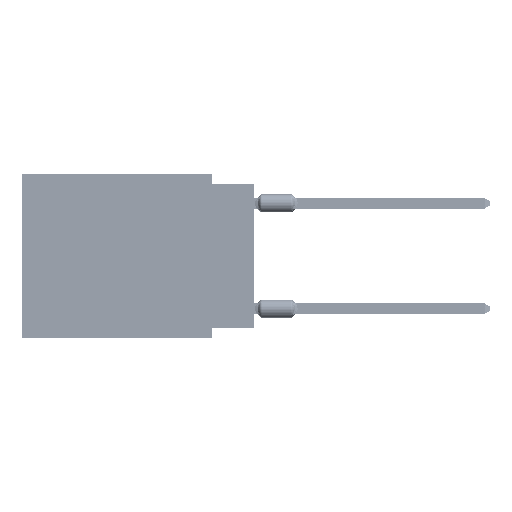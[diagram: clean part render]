
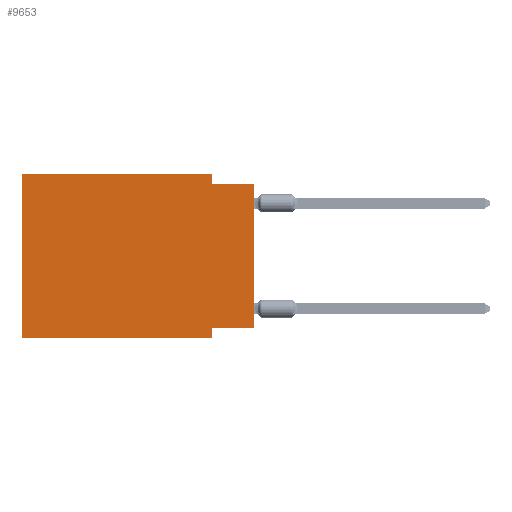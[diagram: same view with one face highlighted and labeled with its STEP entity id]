
A CAD part, left-side view. The second image highlights one B-rep face of the part: STEP entity #9653.
In plain terms, the highlighted planar face has unit normal (-1, 0, 0).
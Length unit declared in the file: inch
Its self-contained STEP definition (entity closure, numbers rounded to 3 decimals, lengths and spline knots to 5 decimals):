
#1042 = PLANE ( 'NONE',  #41379 ) ;
#1323 = LINE ( 'NONE', #72326, #17636 ) ;
#2230 = VECTOR ( 'NONE', #40724, 39.37008 ) ;
#2346 = VERTEX_POINT ( 'NONE', #14057 ) ;
#6202 = ORIENTED_EDGE ( 'NONE', *, *, #41951, .F. ) ;
#7195 = LINE ( 'NONE', #78625, #16957 ) ;
#7771 = VERTEX_POINT ( 'NONE', #80201 ) ;
#7961 = LINE ( 'NONE', #38356, #2230 ) ;
#8092 = VERTEX_POINT ( 'NONE', #33844 ) ;
#9653 = ADVANCED_FACE ( 'NONE', ( #72862 ), #1042, .F. ) ;
#11937 = VERTEX_POINT ( 'NONE', #57361 ) ;
#12796 = LINE ( 'NONE', #76288, #73460 ) ;
#13601 = EDGE_CURVE ( 'NONE', #22929, #8092, #1323, .T. ) ;
#14057 = CARTESIAN_POINT ( 'NONE',  ( 0., 0.55, 0. ) ) ;
#15280 = CARTESIAN_POINT ( 'NONE',  ( 0., 0.55, 0. ) ) ;
#15868 = CARTESIAN_POINT ( 'NONE',  ( 0., 0.1, -0.39 ) ) ;
#16957 = VECTOR ( 'NONE', #77391, 39.37008 ) ;
#17636 = VECTOR ( 'NONE', #26919, 39.37008 ) ;
#21873 = LINE ( 'NONE', #29428, #29114 ) ;
#22428 = EDGE_LOOP ( 'NONE', ( #67440, #48752, #23538, #30403, #28441, #42413, #27757, #6202 ) ) ;
#22727 = VERTEX_POINT ( 'NONE', #46917 ) ;
#22929 = VERTEX_POINT ( 'NONE', #25560 ) ;
#23538 = ORIENTED_EDGE ( 'NONE', *, *, #61757, .F. ) ;
#24059 = LINE ( 'NONE', #50974, #32996 ) ;
#25560 = CARTESIAN_POINT ( 'NONE',  ( 0., 0., -0.365 ) ) ;
#26069 = VECTOR ( 'NONE', #76416, 39.37008 ) ;
#26919 = DIRECTION ( 'NONE',  ( 0., 0., 1. ) ) ;
#27757 = ORIENTED_EDGE ( 'NONE', *, *, #44434, .F. ) ;
#28441 = ORIENTED_EDGE ( 'NONE', *, *, #57004, .F. ) ;
#29114 = VECTOR ( 'NONE', #36160, 39.37008 ) ;
#29428 = CARTESIAN_POINT ( 'NONE',  ( 0., 0.55, 0. ) ) ;
#29948 = VERTEX_POINT ( 'NONE', #15868 ) ;
#30403 = ORIENTED_EDGE ( 'NONE', *, *, #68373, .F. ) ;
#32996 = VECTOR ( 'NONE', #81661, 39.37008 ) ;
#33844 = CARTESIAN_POINT ( 'NONE',  ( 0., 0., -0.025 ) ) ;
#36160 = DIRECTION ( 'NONE',  ( 0., 0., 1. ) ) ;
#38356 = CARTESIAN_POINT ( 'NONE',  ( 0., 0.1, -0.39 ) ) ;
#38652 = DIRECTION ( 'NONE',  ( 0., 0., -1. ) ) ;
#39244 = DIRECTION ( 'NONE',  ( 0., 0., -1. ) ) ;
#40724 = DIRECTION ( 'NONE',  ( 0., 0., -1. ) ) ;
#40921 = DIRECTION ( 'NONE',  ( 1., 0., 0. ) ) ;
#41379 = AXIS2_PLACEMENT_3D ( 'NONE', #15280, #40921, #39244 ) ;
#41951 = EDGE_CURVE ( 'NONE', #22929, #11937, #57927, .T. ) ;
#42413 = ORIENTED_EDGE ( 'NONE', *, *, #77647, .T. ) ;
#44434 = EDGE_CURVE ( 'NONE', #11937, #29948, #7961, .T. ) ;
#46917 = CARTESIAN_POINT ( 'NONE',  ( 0., 0.55, -0.39 ) ) ;
#48752 = ORIENTED_EDGE ( 'NONE', *, *, #55734, .F. ) ;
#50974 = CARTESIAN_POINT ( 'NONE',  ( 0., 0.55, -0.39 ) ) ;
#55734 = EDGE_CURVE ( 'NONE', #58728, #8092, #7195, .T. ) ;
#57004 = EDGE_CURVE ( 'NONE', #22727, #2346, #21873, .T. ) ;
#57361 = CARTESIAN_POINT ( 'NONE',  ( 0., 0.1, -0.365 ) ) ;
#57927 = LINE ( 'NONE', #69706, #26069 ) ;
#58431 = CARTESIAN_POINT ( 'NONE',  ( 0., 0.1, 0. ) ) ;
#58728 = VERTEX_POINT ( 'NONE', #67381 ) ;
#61757 = EDGE_CURVE ( 'NONE', #7771, #58728, #82816, .T. ) ;
#67381 = CARTESIAN_POINT ( 'NONE',  ( 0., 0.1, -0.025 ) ) ;
#67440 = ORIENTED_EDGE ( 'NONE', *, *, #13601, .T. ) ;
#68373 = EDGE_CURVE ( 'NONE', #2346, #7771, #12796, .T. ) ;
#69706 = CARTESIAN_POINT ( 'NONE',  ( 0., 0., -0.365 ) ) ;
#72326 = CARTESIAN_POINT ( 'NONE',  ( 0., 0., 0. ) ) ;
#72862 = FACE_OUTER_BOUND ( 'NONE', #22428, .T. ) ;
#73460 = VECTOR ( 'NONE', #75876, 39.37008 ) ;
#75876 = DIRECTION ( 'NONE',  ( 0., -1., 0. ) ) ;
#76288 = CARTESIAN_POINT ( 'NONE',  ( 0., 0.55, 0. ) ) ;
#76416 = DIRECTION ( 'NONE',  ( 0., 1., 0. ) ) ;
#77391 = DIRECTION ( 'NONE',  ( 0., -1., 0. ) ) ;
#77647 = EDGE_CURVE ( 'NONE', #22727, #29948, #24059, .T. ) ;
#78625 = CARTESIAN_POINT ( 'NONE',  ( 0., 0., -0.025 ) ) ;
#80189 = VECTOR ( 'NONE', #38652, 39.37008 ) ;
#80201 = CARTESIAN_POINT ( 'NONE',  ( 0., 0.1, 0. ) ) ;
#81661 = DIRECTION ( 'NONE',  ( 0., -1., 0. ) ) ;
#82816 = LINE ( 'NONE', #58431, #80189 ) ;
